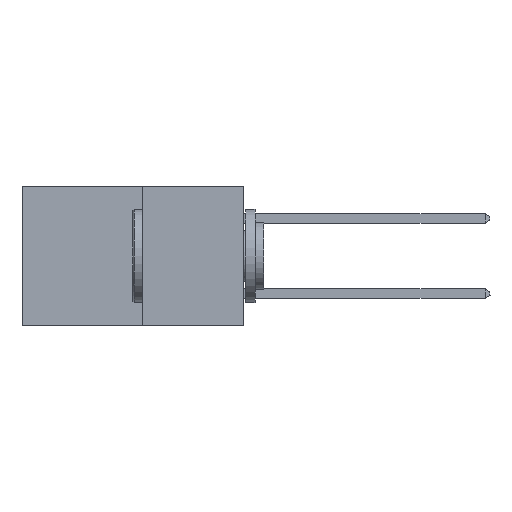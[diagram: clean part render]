
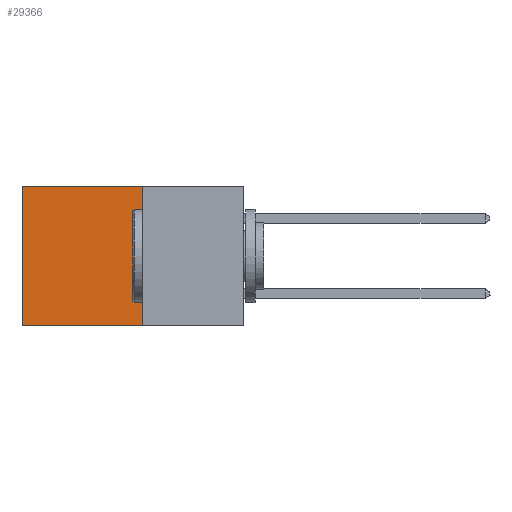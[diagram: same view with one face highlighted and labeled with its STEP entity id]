
A CAD part, left-side view. The second image highlights one B-rep face of the part: STEP entity #29366.
In plain terms, the highlighted planar face has unit normal (-1, 0, 0).
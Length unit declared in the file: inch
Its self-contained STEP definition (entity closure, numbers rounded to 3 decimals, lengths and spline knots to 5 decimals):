
#586 = ORIENTED_EDGE ( 'NONE', *, *, #16646, .F. ) ;
#812 = CARTESIAN_POINT ( 'NONE',  ( 0.277, 0.27, -0.37 ) ) ;
#1626 = CARTESIAN_POINT ( 'NONE',  ( 0.277, 0.27, 0. ) ) ;
#1852 = DIRECTION ( 'NONE',  ( 0., 1., 0. ) ) ;
#2053 = VERTEX_POINT ( 'NONE', #18721 ) ;
#2735 = LINE ( 'NONE', #1626, #26917 ) ;
#3202 = CARTESIAN_POINT ( 'NONE',  ( 0.277, 0.27, -0.37 ) ) ;
#3594 = ORIENTED_EDGE ( 'NONE', *, *, #30385, .T. ) ;
#4607 = CARTESIAN_POINT ( 'NONE',  ( 0.277, 0.59, 0. ) ) ;
#6478 = VECTOR ( 'NONE', #25127, 39.37008 ) ;
#6763 = CARTESIAN_POINT ( 'NONE',  ( 0.277, 0.59, -0.37 ) ) ;
#8156 = EDGE_LOOP ( 'NONE', ( #3594, #23333, #586, #23043 ) ) ;
#8798 = LINE ( 'NONE', #3202, #21774 ) ;
#8874 = EDGE_CURVE ( 'NONE', #2053, #10898, #27830, .T. ) ;
#9113 = FACE_OUTER_BOUND ( 'NONE', #8156, .T. ) ;
#10898 = VERTEX_POINT ( 'NONE', #6763 ) ;
#12904 = DIRECTION ( 'NONE',  ( 0., 0., -1. ) ) ;
#13654 = LINE ( 'NONE', #26445, #6478 ) ;
#13853 = VERTEX_POINT ( 'NONE', #26056 ) ;
#16646 = EDGE_CURVE ( 'NONE', #13853, #2053, #8798, .T. ) ;
#18290 = EDGE_CURVE ( 'NONE', #13853, #29097, #2735, .T. ) ;
#18721 = CARTESIAN_POINT ( 'NONE',  ( 0.277, 0.27, -0.37 ) ) ;
#20138 = DIRECTION ( 'NONE',  ( 0., 0., -1. ) ) ;
#20237 = AXIS2_PLACEMENT_3D ( 'NONE', #812, #27422, #12904 ) ;
#21774 = VECTOR ( 'NONE', #20138, 39.37008 ) ;
#22624 = PLANE ( 'NONE',  #20237 ) ;
#23043 = ORIENTED_EDGE ( 'NONE', *, *, #18290, .T. ) ;
#23333 = ORIENTED_EDGE ( 'NONE', *, *, #8874, .F. ) ;
#25127 = DIRECTION ( 'NONE',  ( 0., 0., -1. ) ) ;
#25840 = DIRECTION ( 'NONE',  ( 0., 1., 0. ) ) ;
#26056 = CARTESIAN_POINT ( 'NONE',  ( 0.277, 0.27, 0. ) ) ;
#26445 = CARTESIAN_POINT ( 'NONE',  ( 0.277, 0.59, -0.37 ) ) ;
#26917 = VECTOR ( 'NONE', #25840, 39.37008 ) ;
#27073 = VECTOR ( 'NONE', #1852, 39.37008 ) ;
#27422 = DIRECTION ( 'NONE',  ( 1., 0., 0. ) ) ;
#27830 = LINE ( 'NONE', #30730, #27073 ) ;
#29097 = VERTEX_POINT ( 'NONE', #4607 ) ;
#29366 = ADVANCED_FACE ( 'NONE', ( #9113 ), #22624, .F. ) ;
#30385 = EDGE_CURVE ( 'NONE', #29097, #10898, #13654, .T. ) ;
#30730 = CARTESIAN_POINT ( 'NONE',  ( 0.277, 0.27, -0.37 ) ) ;
